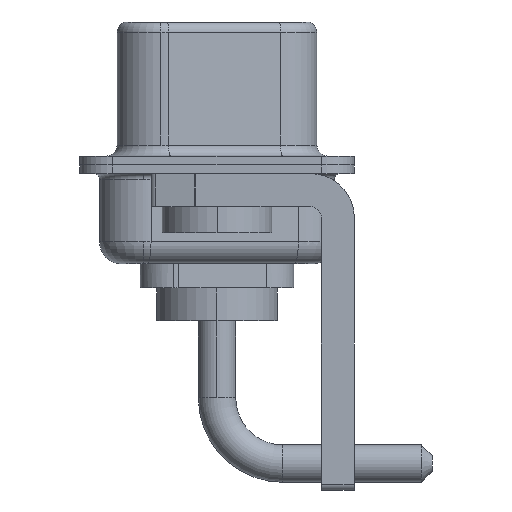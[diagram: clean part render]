
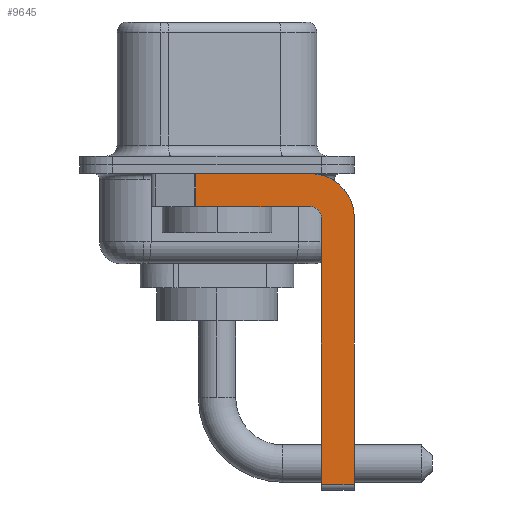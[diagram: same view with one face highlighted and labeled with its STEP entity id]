
A CAD part, left-side view. The second image highlights one B-rep face of the part: STEP entity #9645.
In plain terms, the highlighted planar face has unit normal (-1, 0, 0).
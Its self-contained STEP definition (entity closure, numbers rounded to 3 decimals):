
#40 = CARTESIAN_POINT ( 'NONE',  ( -2.9, -4.25, -1.9 ) ) ;
#332 = EDGE_CURVE ( 'NONE', #6132, #5803, #7562, .T. ) ;
#643 = AXIS2_PLACEMENT_3D ( 'NONE', #5448, #3250, #8413 ) ;
#1269 = EDGE_CURVE ( 'NONE', #9956, #7724, #13473, .T. ) ;
#1904 = FACE_OUTER_BOUND ( 'NONE', #6817, .T. ) ;
#3250 = DIRECTION ( 'NONE',  ( 1., 0., 0. ) ) ;
#3303 = CARTESIAN_POINT ( 'NONE',  ( -2.9, -6.25, -2.4 ) ) ;
#3378 = DIRECTION ( 'NONE',  ( 0., 0., 1. ) ) ;
#3639 = VECTOR ( 'NONE', #13530, 1000. ) ;
#3923 = CARTESIAN_POINT ( 'NONE',  ( -2.9, -4.25, -0.4 ) ) ;
#4107 = CARTESIAN_POINT ( 'NONE',  ( -2.9, -4.25, -2.4 ) ) ;
#4416 = DIRECTION ( 'NONE',  ( 0., -1., 0. ) ) ;
#4526 = PLANE ( 'NONE',  #643 ) ;
#4586 = CARTESIAN_POINT ( 'NONE',  ( -2.9, -4.75, -14.55 ) ) ;
#5096 = DIRECTION ( 'NONE',  ( 0., -1., 0. ) ) ;
#5102 = CARTESIAN_POINT ( 'NONE',  ( -2.9, -6.25, -14.55 ) ) ;
#5412 = EDGE_CURVE ( 'NONE', #7517, #11779, #15264, .T. ) ;
#5448 = CARTESIAN_POINT ( 'NONE',  ( -2.9, -4.25, -2.4 ) ) ;
#5603 = EDGE_CURVE ( 'NONE', #11779, #11624, #8577, .T. ) ;
#5713 = CARTESIAN_POINT ( 'NONE',  ( -2.9, 0.978, -1.9 ) ) ;
#5803 = VERTEX_POINT ( 'NONE', #5102 ) ;
#6083 = EDGE_CURVE ( 'NONE', #7724, #5803, #9809, .T. ) ;
#6132 = VERTEX_POINT ( 'NONE', #4586 ) ;
#6165 = CARTESIAN_POINT ( 'NONE',  ( -2.9, 0.978, -0.4 ) ) ;
#6718 = VECTOR ( 'NONE', #3378, 1000. ) ;
#6817 = EDGE_LOOP ( 'NONE', ( #10012, #15119, #14311, #9995, #12114, #9774, #7583, #8211 ) ) ;
#7126 = DIRECTION ( 'NONE',  ( 0., 0., -1. ) ) ;
#7517 = VERTEX_POINT ( 'NONE', #12583 ) ;
#7562 = LINE ( 'NONE', #11657, #7581 ) ;
#7581 = VECTOR ( 'NONE', #5096, 1000. ) ;
#7583 = ORIENTED_EDGE ( 'NONE', *, *, #6083, .F. ) ;
#7724 = VERTEX_POINT ( 'NONE', #10550 ) ;
#8211 = ORIENTED_EDGE ( 'NONE', *, *, #1269, .F. ) ;
#8413 = DIRECTION ( 'NONE',  ( 0., 0., -1. ) ) ;
#8449 = CARTESIAN_POINT ( 'NONE',  ( -2.9, -4.75, -14.8 ) ) ;
#8577 = LINE ( 'NONE', #9580, #9410 ) ;
#9410 = VECTOR ( 'NONE', #14859, 1000. ) ;
#9580 = CARTESIAN_POINT ( 'NONE',  ( -2.9, -4.25, -1.9 ) ) ;
#9645 = ADVANCED_FACE ( 'NONE', ( #1904 ), #4526, .F. ) ;
#9774 = ORIENTED_EDGE ( 'NONE', *, *, #332, .T. ) ;
#9809 = LINE ( 'NONE', #3303, #13169 ) ;
#9956 = VERTEX_POINT ( 'NONE', #3923 ) ;
#9994 = AXIS2_PLACEMENT_3D ( 'NONE', #15288, #11759, #12705 ) ;
#9995 = ORIENTED_EDGE ( 'NONE', *, *, #5412, .F. ) ;
#10012 = ORIENTED_EDGE ( 'NONE', *, *, #13011, .F. ) ;
#10550 = CARTESIAN_POINT ( 'NONE',  ( -2.9, -6.25, -2.4 ) ) ;
#10948 = EDGE_CURVE ( 'NONE', #15178, #11624, #12183, .T. ) ;
#11624 = VERTEX_POINT ( 'NONE', #12587 ) ;
#11657 = CARTESIAN_POINT ( 'NONE',  ( -2.9, -4.25, -14.55 ) ) ;
#11759 = DIRECTION ( 'NONE',  ( 1., 0., 0. ) ) ;
#11779 = VERTEX_POINT ( 'NONE', #40 ) ;
#11922 = DIRECTION ( 'NONE',  ( 0., 0., 1. ) ) ;
#12114 = ORIENTED_EDGE ( 'NONE', *, *, #16407, .F. ) ;
#12156 = CARTESIAN_POINT ( 'NONE',  ( -2.9, 3., -0.4 ) ) ;
#12183 = LINE ( 'NONE', #5713, #3639 ) ;
#12475 = LINE ( 'NONE', #8449, #6718 ) ;
#12583 = CARTESIAN_POINT ( 'NONE',  ( -2.9, -4.75, -2.4 ) ) ;
#12587 = CARTESIAN_POINT ( 'NONE',  ( -2.9, 0.978, -1.9 ) ) ;
#12705 = DIRECTION ( 'NONE',  ( 0., 0., -1. ) ) ;
#13011 = EDGE_CURVE ( 'NONE', #15178, #9956, #13753, .T. ) ;
#13169 = VECTOR ( 'NONE', #7126, 1000. ) ;
#13473 = CIRCLE ( 'NONE', #9994, 2. ) ;
#13530 = DIRECTION ( 'NONE',  ( 0., 0., -1. ) ) ;
#13753 = LINE ( 'NONE', #12156, #13929 ) ;
#13929 = VECTOR ( 'NONE', #4416, 1000. ) ;
#14311 = ORIENTED_EDGE ( 'NONE', *, *, #5603, .F. ) ;
#14859 = DIRECTION ( 'NONE',  ( 0., 1., 0. ) ) ;
#15119 = ORIENTED_EDGE ( 'NONE', *, *, #10948, .T. ) ;
#15178 = VERTEX_POINT ( 'NONE', #6165 ) ;
#15264 = CIRCLE ( 'NONE', #16623, 0.5 ) ;
#15288 = CARTESIAN_POINT ( 'NONE',  ( -2.9, -4.25, -2.4 ) ) ;
#15869 = DIRECTION ( 'NONE',  ( -1., 0., 0. ) ) ;
#16407 = EDGE_CURVE ( 'NONE', #6132, #7517, #12475, .T. ) ;
#16623 = AXIS2_PLACEMENT_3D ( 'NONE', #4107, #15869, #11922 ) ;
